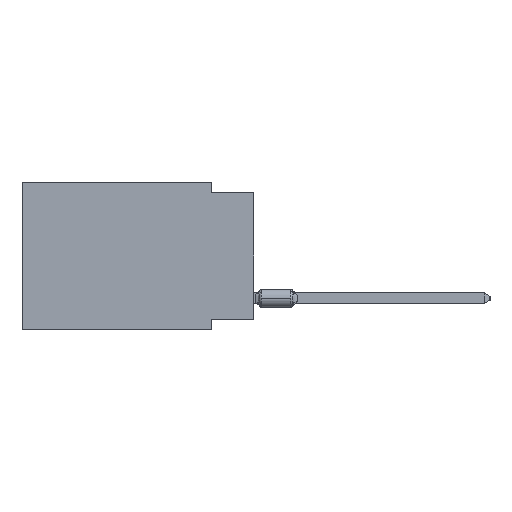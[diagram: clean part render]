
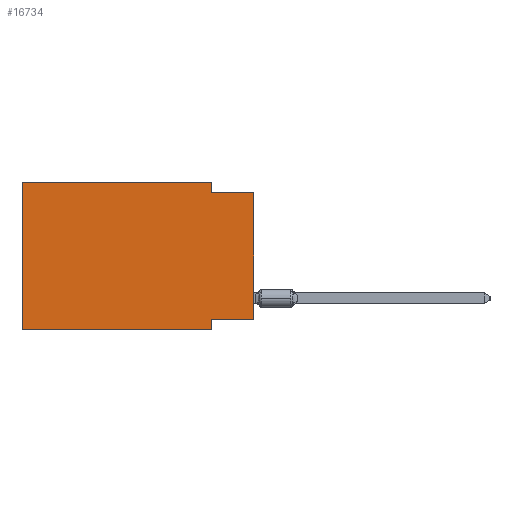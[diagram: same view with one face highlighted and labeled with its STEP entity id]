
A CAD part, left-side view. The second image highlights one B-rep face of the part: STEP entity #16734.
In plain terms, the highlighted planar face has unit normal (-1, 0, 0).
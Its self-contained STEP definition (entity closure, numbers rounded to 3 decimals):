
#450 = ORIENTED_EDGE ( 'NONE', *, *, #14038, .T. ) ;
#1973 = LINE ( 'NONE', #42456, #94867 ) ;
#4336 = ORIENTED_EDGE ( 'NONE', *, *, #60177, .T. ) ;
#6020 = CARTESIAN_POINT ( 'NONE',  ( 0., 13.97, 0. ) ) ;
#7419 = LINE ( 'NONE', #55694, #58501 ) ;
#8212 = VERTEX_POINT ( 'NONE', #6020 ) ;
#8724 = ORIENTED_EDGE ( 'NONE', *, *, #47918, .F. ) ;
#11337 = VERTEX_POINT ( 'NONE', #20150 ) ;
#11984 = VECTOR ( 'NONE', #84012, 1000. ) ;
#14038 = EDGE_CURVE ( 'NONE', #57160, #71247, #87908, .T. ) ;
#15986 = EDGE_LOOP ( 'NONE', ( #4336, #77887, #8724, #81858, #86174, #450, #68117, #59805 ) ) ;
#16734 = ADVANCED_FACE ( 'NONE', ( #57496 ), #18031, .F. ) ;
#18031 = PLANE ( 'NONE',  #56130 ) ;
#18586 = CARTESIAN_POINT ( 'NONE',  ( 0., 2.54, 0. ) ) ;
#18885 = VECTOR ( 'NONE', #54621, 1000. ) ;
#19879 = CARTESIAN_POINT ( 'NONE',  ( 0., 0., -8.255 ) ) ;
#20150 = CARTESIAN_POINT ( 'NONE',  ( 0., 2.54, -0.635 ) ) ;
#22005 = VECTOR ( 'NONE', #89891, 1000. ) ;
#22646 = EDGE_CURVE ( 'NONE', #57160, #8212, #62921, .T. ) ;
#25227 = VECTOR ( 'NONE', #42235, 1000. ) ;
#26327 = VERTEX_POINT ( 'NONE', #18586 ) ;
#27986 = CARTESIAN_POINT ( 'NONE',  ( 0., 0., -8.255 ) ) ;
#29706 = CARTESIAN_POINT ( 'NONE',  ( 0., 13.97, 0. ) ) ;
#30966 = CARTESIAN_POINT ( 'NONE',  ( 0., 13.97, -8.89 ) ) ;
#32899 = CARTESIAN_POINT ( 'NONE',  ( 0., 13.97, -8.89 ) ) ;
#34426 = DIRECTION ( 'NONE',  ( 0., -1., 0. ) ) ;
#34624 = CARTESIAN_POINT ( 'NONE',  ( 0., 2.54, -8.89 ) ) ;
#36655 = DIRECTION ( 'NONE',  ( 1., 0., 0. ) ) ;
#39540 = EDGE_CURVE ( 'NONE', #8212, #26327, #60091, .T. ) ;
#39604 = DIRECTION ( 'NONE',  ( 0., 0., -1. ) ) ;
#42235 = DIRECTION ( 'NONE',  ( 0., -1., 0. ) ) ;
#42456 = CARTESIAN_POINT ( 'NONE',  ( 0., 0., 0. ) ) ;
#42735 = LINE ( 'NONE', #80119, #25227 ) ;
#47918 = EDGE_CURVE ( 'NONE', #26327, #11337, #74331, .T. ) ;
#48926 = EDGE_CURVE ( 'NONE', #11337, #56474, #42735, .T. ) ;
#49711 = CARTESIAN_POINT ( 'NONE',  ( 0., 13.97, 0. ) ) ;
#50388 = CARTESIAN_POINT ( 'NONE',  ( 0., 0., -0.635 ) ) ;
#54621 = DIRECTION ( 'NONE',  ( 0., 0., 1. ) ) ;
#55667 = VECTOR ( 'NONE', #67377, 1000. ) ;
#55694 = CARTESIAN_POINT ( 'NONE',  ( 0., 2.54, -8.89 ) ) ;
#56130 = AXIS2_PLACEMENT_3D ( 'NONE', #49711, #36655, #83869 ) ;
#56474 = VERTEX_POINT ( 'NONE', #50388 ) ;
#57160 = VERTEX_POINT ( 'NONE', #30966 ) ;
#57496 = FACE_OUTER_BOUND ( 'NONE', #15986, .T. ) ;
#58501 = VECTOR ( 'NONE', #39604, 1000. ) ;
#59805 = ORIENTED_EDGE ( 'NONE', *, *, #69134, .F. ) ;
#60091 = LINE ( 'NONE', #74142, #55667 ) ;
#60177 = EDGE_CURVE ( 'NONE', #78171, #56474, #1973, .T. ) ;
#62921 = LINE ( 'NONE', #29706, #18885 ) ;
#66829 = DIRECTION ( 'NONE',  ( 0., 0., 1. ) ) ;
#67377 = DIRECTION ( 'NONE',  ( 0., -1., 0. ) ) ;
#68117 = ORIENTED_EDGE ( 'NONE', *, *, #70602, .F. ) ;
#69134 = EDGE_CURVE ( 'NONE', #78171, #99928, #99585, .T. ) ;
#70602 = EDGE_CURVE ( 'NONE', #99928, #71247, #7419, .T. ) ;
#71247 = VERTEX_POINT ( 'NONE', #34624 ) ;
#71367 = CARTESIAN_POINT ( 'NONE',  ( 0., 2.54, -8.255 ) ) ;
#74142 = CARTESIAN_POINT ( 'NONE',  ( 0., 13.97, 0. ) ) ;
#74331 = LINE ( 'NONE', #96673, #22005 ) ;
#77887 = ORIENTED_EDGE ( 'NONE', *, *, #48926, .F. ) ;
#78171 = VERTEX_POINT ( 'NONE', #19879 ) ;
#80119 = CARTESIAN_POINT ( 'NONE',  ( 0., 0., -0.635 ) ) ;
#81858 = ORIENTED_EDGE ( 'NONE', *, *, #39540, .F. ) ;
#83869 = DIRECTION ( 'NONE',  ( 0., 0., -1. ) ) ;
#84012 = DIRECTION ( 'NONE',  ( 0., 1., 0. ) ) ;
#86174 = ORIENTED_EDGE ( 'NONE', *, *, #22646, .F. ) ;
#87908 = LINE ( 'NONE', #32899, #89180 ) ;
#89180 = VECTOR ( 'NONE', #34426, 1000. ) ;
#89891 = DIRECTION ( 'NONE',  ( 0., 0., -1. ) ) ;
#94867 = VECTOR ( 'NONE', #66829, 1000. ) ;
#96673 = CARTESIAN_POINT ( 'NONE',  ( 0., 2.54, 0. ) ) ;
#99585 = LINE ( 'NONE', #27986, #11984 ) ;
#99928 = VERTEX_POINT ( 'NONE', #71367 ) ;
